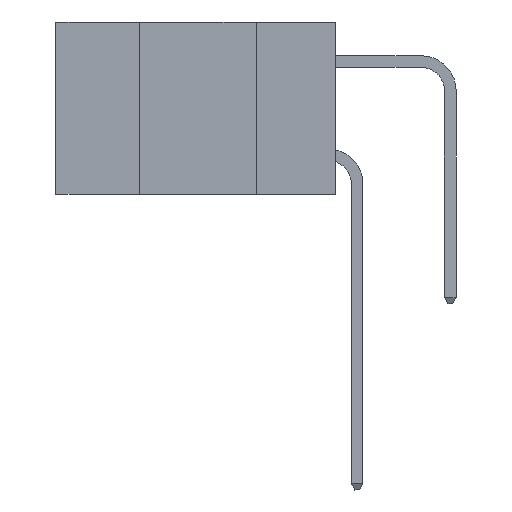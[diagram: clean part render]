
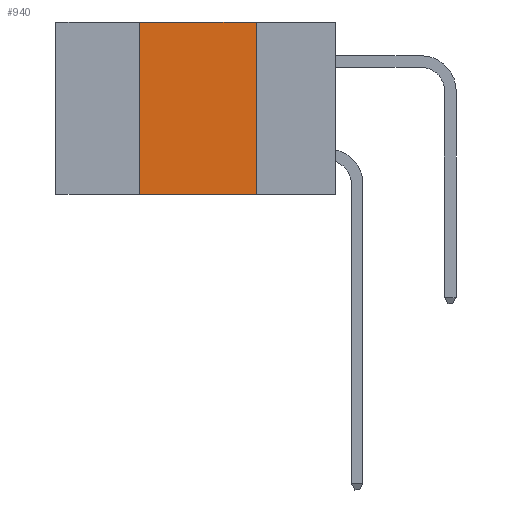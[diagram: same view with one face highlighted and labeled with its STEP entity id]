
A CAD part, left-side view. The second image highlights one B-rep face of the part: STEP entity #940.
In plain terms, the highlighted planar face has unit normal (-1, 0, 0).
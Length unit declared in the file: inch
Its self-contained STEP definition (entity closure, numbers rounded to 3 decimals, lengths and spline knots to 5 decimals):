
#332 = VERTEX_POINT ( 'NONE', #3969 ) ;
#341 = CARTESIAN_POINT ( 'NONE',  ( 0., 0.42, 0. ) ) ;
#940 = ADVANCED_FACE ( 'NONE', ( #14773 ), #3246, .F. ) ;
#986 = ORIENTED_EDGE ( 'NONE', *, *, #7736, .F. ) ;
#1781 = CARTESIAN_POINT ( 'NONE',  ( 0., 0.17, 0. ) ) ;
#2044 = VERTEX_POINT ( 'NONE', #5607 ) ;
#2774 = DIRECTION ( 'NONE',  ( 0., -1., 0. ) ) ;
#3127 = DIRECTION ( 'NONE',  ( 0., -1., 0. ) ) ;
#3246 = PLANE ( 'NONE',  #9681 ) ;
#3598 = CARTESIAN_POINT ( 'NONE',  ( 0., 0.6, -0.37 ) ) ;
#3603 = EDGE_CURVE ( 'NONE', #9069, #2044, #3659, .T. ) ;
#3659 = LINE ( 'NONE', #3598, #16075 ) ;
#3969 = CARTESIAN_POINT ( 'NONE',  ( 0., 0.42, 0. ) ) ;
#4147 = LINE ( 'NONE', #341, #14778 ) ;
#4995 = VERTEX_POINT ( 'NONE', #10308 ) ;
#5151 = VECTOR ( 'NONE', #2774, 39.37008 ) ;
#5607 = CARTESIAN_POINT ( 'NONE',  ( 0., 0.17, -0.37 ) ) ;
#6145 = DIRECTION ( 'NONE',  ( 1., 0., 0. ) ) ;
#6189 = DIRECTION ( 'NONE',  ( 0., 0., 1. ) ) ;
#6784 = ORIENTED_EDGE ( 'NONE', *, *, #14537, .F. ) ;
#7202 = LINE ( 'NONE', #1781, #13033 ) ;
#7464 = EDGE_LOOP ( 'NONE', ( #10226, #986, #6784, #7980 ) ) ;
#7736 = EDGE_CURVE ( 'NONE', #332, #4995, #8560, .T. ) ;
#7980 = ORIENTED_EDGE ( 'NONE', *, *, #3603, .T. ) ;
#8048 = DIRECTION ( 'NONE',  ( 0., 0., -1. ) ) ;
#8560 = LINE ( 'NONE', #14185, #5151 ) ;
#9069 = VERTEX_POINT ( 'NONE', #13316 ) ;
#9681 = AXIS2_PLACEMENT_3D ( 'NONE', #13494, #6145, #15104 ) ;
#10226 = ORIENTED_EDGE ( 'NONE', *, *, #12196, .F. ) ;
#10308 = CARTESIAN_POINT ( 'NONE',  ( 0., 0.17, 0. ) ) ;
#12196 = EDGE_CURVE ( 'NONE', #4995, #2044, #7202, .T. ) ;
#13033 = VECTOR ( 'NONE', #8048, 39.37008 ) ;
#13316 = CARTESIAN_POINT ( 'NONE',  ( 0., 0.42, -0.37 ) ) ;
#13494 = CARTESIAN_POINT ( 'NONE',  ( 0., 0.6, 0. ) ) ;
#14185 = CARTESIAN_POINT ( 'NONE',  ( 0., 0.6, 0. ) ) ;
#14537 = EDGE_CURVE ( 'NONE', #9069, #332, #4147, .T. ) ;
#14773 = FACE_OUTER_BOUND ( 'NONE', #7464, .T. ) ;
#14778 = VECTOR ( 'NONE', #6189, 39.37008 ) ;
#15104 = DIRECTION ( 'NONE',  ( 0., 0., -1. ) ) ;
#16075 = VECTOR ( 'NONE', #3127, 39.37008 ) ;
